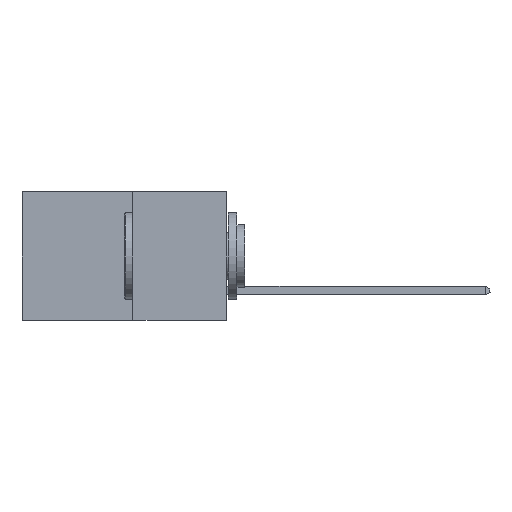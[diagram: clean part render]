
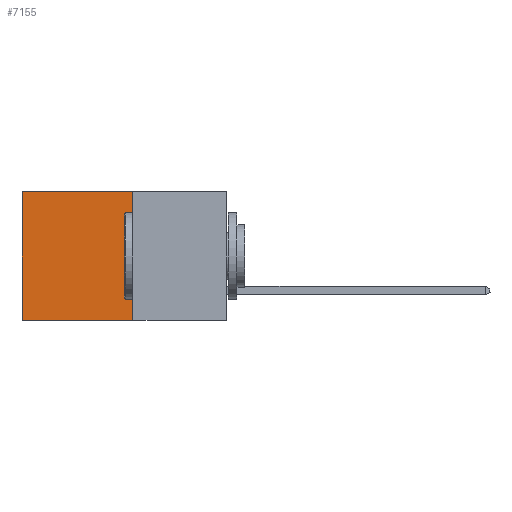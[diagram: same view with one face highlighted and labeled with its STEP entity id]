
A CAD part, left-side view. The second image highlights one B-rep face of the part: STEP entity #7155.
In plain terms, the highlighted planar face has unit normal (-1, 0, 0).
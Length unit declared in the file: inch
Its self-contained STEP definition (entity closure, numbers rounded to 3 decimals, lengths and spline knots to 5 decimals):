
#16 = CARTESIAN_POINT ( 'NONE',  ( 0.277, 0.27, 0. ) ) ;
#498 = LINE ( 'NONE', #16, #6332 ) ;
#858 = EDGE_CURVE ( 'NONE', #10080, #7744, #4584, .T. ) ;
#1076 = ORIENTED_EDGE ( 'NONE', *, *, #1906, .F. ) ;
#1868 = VECTOR ( 'NONE', #13262, 39.37008 ) ;
#1906 = EDGE_CURVE ( 'NONE', #4091, #10080, #5610, .T. ) ;
#1992 = DIRECTION ( 'NONE',  ( 0., 0., -1. ) ) ;
#2642 = ORIENTED_EDGE ( 'NONE', *, *, #13075, .T. ) ;
#2831 = EDGE_LOOP ( 'NONE', ( #7520, #7699, #1076, #2642 ) ) ;
#3271 = CARTESIAN_POINT ( 'NONE',  ( 0.277, 0.27, -0.37 ) ) ;
#3319 = LINE ( 'NONE', #10435, #6071 ) ;
#4091 = VERTEX_POINT ( 'NONE', #10823 ) ;
#4248 = CARTESIAN_POINT ( 'NONE',  ( 0.277, 0.27, -0.37 ) ) ;
#4584 = LINE ( 'NONE', #3271, #1868 ) ;
#4846 = EDGE_CURVE ( 'NONE', #12174, #7744, #3319, .T. ) ;
#5280 = DIRECTION ( 'NONE',  ( 1., 0., 0. ) ) ;
#5304 = VECTOR ( 'NONE', #7512, 39.37008 ) ;
#5610 = LINE ( 'NONE', #7430, #5304 ) ;
#6071 = VECTOR ( 'NONE', #1992, 39.37008 ) ;
#6332 = VECTOR ( 'NONE', #7611, 39.37008 ) ;
#7155 = ADVANCED_FACE ( 'NONE', ( #8512 ), #10163, .F. ) ;
#7430 = CARTESIAN_POINT ( 'NONE',  ( 0.277, 0.27, -0.37 ) ) ;
#7512 = DIRECTION ( 'NONE',  ( 0., 0., -1. ) ) ;
#7520 = ORIENTED_EDGE ( 'NONE', *, *, #4846, .T. ) ;
#7611 = DIRECTION ( 'NONE',  ( 0., 1., 0. ) ) ;
#7699 = ORIENTED_EDGE ( 'NONE', *, *, #858, .F. ) ;
#7744 = VERTEX_POINT ( 'NONE', #7877 ) ;
#7877 = CARTESIAN_POINT ( 'NONE',  ( 0.277, 0.59, -0.37 ) ) ;
#8256 = AXIS2_PLACEMENT_3D ( 'NONE', #4248, #5280, #12122 ) ;
#8512 = FACE_OUTER_BOUND ( 'NONE', #2831, .T. ) ;
#10080 = VERTEX_POINT ( 'NONE', #10345 ) ;
#10163 = PLANE ( 'NONE',  #8256 ) ;
#10345 = CARTESIAN_POINT ( 'NONE',  ( 0.277, 0.27, -0.37 ) ) ;
#10435 = CARTESIAN_POINT ( 'NONE',  ( 0.277, 0.59, -0.37 ) ) ;
#10823 = CARTESIAN_POINT ( 'NONE',  ( 0.277, 0.27, 0. ) ) ;
#12122 = DIRECTION ( 'NONE',  ( 0., 0., -1. ) ) ;
#12174 = VERTEX_POINT ( 'NONE', #12463 ) ;
#12463 = CARTESIAN_POINT ( 'NONE',  ( 0.277, 0.59, 0. ) ) ;
#13075 = EDGE_CURVE ( 'NONE', #4091, #12174, #498, .T. ) ;
#13262 = DIRECTION ( 'NONE',  ( 0., 1., 0. ) ) ;
